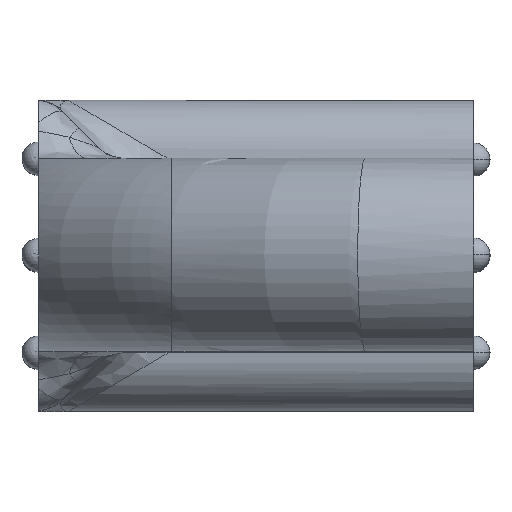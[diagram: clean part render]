
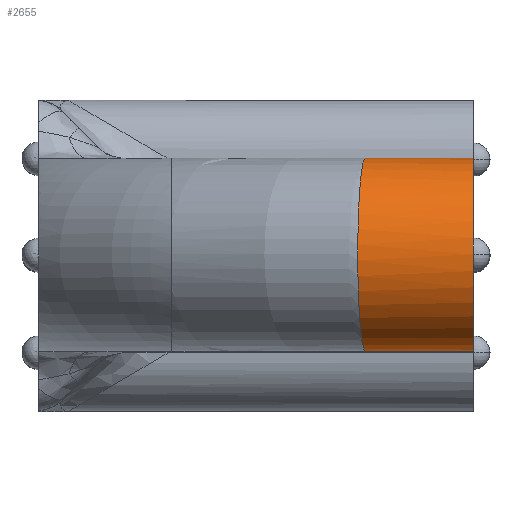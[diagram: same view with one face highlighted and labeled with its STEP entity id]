
A CAD part, top view. The second image highlights one B-rep face of the part: STEP entity #2655.
In plain terms, the highlighted cylindrical face has radius 11.509 mm (diameter 23.019 mm), a partial arc.
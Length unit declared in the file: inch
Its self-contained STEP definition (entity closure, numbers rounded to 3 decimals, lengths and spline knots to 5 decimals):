
#6 = CARTESIAN_POINT ( 'NONE',  ( 2.26457, -0.8937, 0.96371 ) ) ;
#24 = CARTESIAN_POINT ( 'NONE',  ( 1.75888, -0.8937, 0.96371 ) ) ;
#48 = DIRECTION ( 'NONE',  ( -1., 0., 0. ) ) ;
#53 = CARTESIAN_POINT ( 'NONE',  ( 8.36796, -0.8937, 0.96371 ) ) ;
#144 = CIRCLE ( 'NONE', #2152, 0.45313 ) ;
#151 = VECTOR ( 'NONE', #2381, 39.37008 ) ;
#177 = LINE ( 'NONE', #2359, #151 ) ;
#347 = CYLINDRICAL_SURFACE ( 'NONE', #2343, 0.45313 ) ;
#355 = FACE_OUTER_BOUND ( 'NONE', #2465, .T. ) ;
#608 = LINE ( 'NONE', #53, #613 ) ;
#613 = VECTOR ( 'NONE', #48, 39.37008 ) ;
#1392 = CARTESIAN_POINT ( 'NONE',  ( 1.75888, -1.79995, 0.96371 ) ) ;
#1609 = EDGE_CURVE ( 'NONE', #1746, #1688, #608, .T. ) ;
#1688 = VERTEX_POINT ( 'NONE', #24 ) ;
#1746 = VERTEX_POINT ( 'NONE', #6 ) ;
#1852 = VERTEX_POINT ( 'NONE', #3689 ) ;
#1872 = CARTESIAN_POINT ( 'NONE',  ( 1.75888, -1.79995, 0.96371 ) ) ;
#1876 = CARTESIAN_POINT ( 'NONE',  ( 1.75826, -1.79995, 0.97107 ) ) ;
#1880 = CARTESIAN_POINT ( 'NONE',  ( 1.75762, -1.79976, 0.97861 ) ) ;
#1885 = CARTESIAN_POINT ( 'NONE',  ( 1.75636, -1.79903, 0.99351 ) ) ;
#1889 = CARTESIAN_POINT ( 'NONE',  ( 1.75573, -1.79848, 1.00096 ) ) ;
#1890 = CARTESIAN_POINT ( 'NONE',  ( 1.75385, -1.79627, 1.02325 ) ) ;
#1895 = CARTESIAN_POINT ( 'NONE',  ( 1.75262, -1.79407, 1.03793 ) ) ;
#1901 = CARTESIAN_POINT ( 'NONE',  ( 1.74901, -1.7854, 1.08138 ) ) ;
#1902 = CARTESIAN_POINT ( 'NONE',  ( 1.74669, -1.77685, 1.10959 ) ) ;
#1906 = CARTESIAN_POINT ( 'NONE',  ( 1.74333, -1.75981, 1.15074 ) ) ;
#1908 = CARTESIAN_POINT ( 'NONE',  ( 1.74223, -1.75339, 1.16431 ) ) ;
#1915 = CARTESIAN_POINT ( 'NONE',  ( 1.74011, -1.7394, 1.19049 ) ) ;
#1916 = CARTESIAN_POINT ( 'NONE',  ( 1.73909, -1.73179, 1.20316 ) ) ;
#1921 = CARTESIAN_POINT ( 'NONE',  ( 1.73614, -1.70721, 1.23996 ) ) ;
#1922 = CARTESIAN_POINT ( 'NONE',  ( 1.73432, -1.68841, 1.26293 ) ) ;
#1929 = CARTESIAN_POINT ( 'NONE',  ( 1.73098, -1.64615, 1.30521 ) ) ;
#1933 = CARTESIAN_POINT ( 'NONE',  ( 1.72951, -1.62327, 1.32395 ) ) ;
#1935 = CARTESIAN_POINT ( 'NONE',  ( 1.72759, -1.58642, 1.34859 ) ) ;
#1944 = CARTESIAN_POINT ( 'NONE',  ( 1.727, -1.57371, 1.35622 ) ) ;
#1945 = CARTESIAN_POINT ( 'NONE',  ( 1.72591, -1.54742, 1.37029 ) ) ;
#1949 = CARTESIAN_POINT ( 'NONE',  ( 1.72541, -1.53384, 1.37671 ) ) ;
#1952 = CARTESIAN_POINT ( 'NONE',  ( 1.72409, -1.49267, 1.39375 ) ) ;
#1956 = CARTESIAN_POINT ( 'NONE',  ( 1.72343, -1.46439, 1.40232 ) ) ;
#1961 = CARTESIAN_POINT ( 'NONE',  ( 1.72277, -1.42071, 1.41102 ) ) ;
#1962 = CARTESIAN_POINT ( 'NONE',  ( 1.7226, -1.40586, 1.41322 ) ) ;
#1968 = CARTESIAN_POINT ( 'NONE',  ( 1.72237, -1.37614, 1.41613 ) ) ;
#1969 = CARTESIAN_POINT ( 'NONE',  ( 1.72232, -1.36132, 1.41684 ) ) ;
#1974 = CARTESIAN_POINT ( 'NONE',  ( 1.72232, -1.31693, 1.41682 ) ) ;
#1977 = CARTESIAN_POINT ( 'NONE',  ( 1.72254, -1.28748, 1.41393 ) ) ;
#1979 = CARTESIAN_POINT ( 'NONE',  ( 1.72322, -1.24349, 1.40515 ) ) ;
#1983 = CARTESIAN_POINT ( 'NONE',  ( 1.7235, -1.22897, 1.40149 ) ) ;
#1984 = CARTESIAN_POINT ( 'NONE',  ( 1.72416, -1.2006, 1.39285 ) ) ;
#1988 = CARTESIAN_POINT ( 'NONE',  ( 1.72494, -1.17277, 1.38285 ) ) ;
#1990 = CARTESIAN_POINT ( 'NONE',  ( 1.72592, -1.14602, 1.37019 ) ) ;
#1992 = CARTESIAN_POINT ( 'NONE',  ( 1.727, -1.11983, 1.35616 ) ) ;
#1995 = CARTESIAN_POINT ( 'NONE',  ( 1.72761, -1.10694, 1.34842 ) ) ;
#1996 = CARTESIAN_POINT ( 'NONE',  ( 1.72955, -1.06983, 1.32355 ) ) ;
#2001 = CARTESIAN_POINT ( 'NONE',  ( 1.73102, -1.04704, 1.30478 ) ) ;
#2006 = CARTESIAN_POINT ( 'NONE',  ( 1.73432, -1.00525, 1.26292 ) ) ;
#2007 = CARTESIAN_POINT ( 'NONE',  ( 1.73617, -0.98613, 1.23958 ) ) ;
#2010 = CARTESIAN_POINT ( 'NONE',  ( 1.74012, -0.95334, 1.19035 ) ) ;
#2011 = CARTESIAN_POINT ( 'NONE',  ( 1.74222, -0.93945, 1.16434 ) ) ;
#2020 = CARTESIAN_POINT ( 'NONE',  ( 1.74558, -0.92243, 1.12319 ) ) ;
#2022 = CARTESIAN_POINT ( 'NONE',  ( 1.74673, -0.91739, 1.10906 ) ) ;
#2026 = CARTESIAN_POINT ( 'NONE',  ( 1.74907, -0.9088, 1.08065 ) ) ;
#2029 = CARTESIAN_POINT ( 'NONE',  ( 1.75026, -0.90522, 1.06632 ) ) ;
#2036 = CARTESIAN_POINT ( 'NONE',  ( 1.75267, -0.89949, 1.03742 ) ) ;
#2038 = CARTESIAN_POINT ( 'NONE',  ( 1.75389, -0.89733, 1.02284 ) ) ;
#2046 = CARTESIAN_POINT ( 'NONE',  ( 1.75574, -0.89516, 1.0008 ) ) ;
#2049 = CARTESIAN_POINT ( 'NONE',  ( 1.75636, -0.89461, 0.99342 ) ) ;
#2051 = CARTESIAN_POINT ( 'NONE',  ( 1.75762, -0.89388, 0.9786 ) ) ;
#2054 = CARTESIAN_POINT ( 'NONE',  ( 1.75826, -0.8937, 0.97107 ) ) ;
#2057 = CARTESIAN_POINT ( 'NONE',  ( 1.75888, -0.8937, 0.96371 ) ) ;
#2120 = DIRECTION ( 'NONE',  ( 0., -1., 0. ) ) ;
#2123 = DIRECTION ( 'NONE',  ( 1., 0., 0. ) ) ;
#2128 = CARTESIAN_POINT ( 'NONE',  ( 2.26457, -1.34682, 0.96371 ) ) ;
#2152 = AXIS2_PLACEMENT_3D ( 'NONE', #2128, #2123, #2120 ) ;
#2179 = ORIENTED_EDGE ( 'NONE', *, *, #3055, .F. ) ;
#2190 = ORIENTED_EDGE ( 'NONE', *, *, #1609, .T. ) ;
#2202 = ORIENTED_EDGE ( 'NONE', *, *, #3069, .T. ) ;
#2220 = ORIENTED_EDGE ( 'NONE', *, *, #2939, .F. ) ;
#2343 = AXIS2_PLACEMENT_3D ( 'NONE', #2419, #2410, #2402 ) ;
#2359 = CARTESIAN_POINT ( 'NONE',  ( 8.36796, -1.79995, 0.96371 ) ) ;
#2381 = DIRECTION ( 'NONE',  ( -1., 0., 0. ) ) ;
#2402 = DIRECTION ( 'NONE',  ( 0., 1., 0. ) ) ;
#2410 = DIRECTION ( 'NONE',  ( -1., 0., 0. ) ) ;
#2419 = CARTESIAN_POINT ( 'NONE',  ( 8.36796, -1.34682, 0.96371 ) ) ;
#2465 = EDGE_LOOP ( 'NONE', ( #2179, #2190, #2202, #2220 ) ) ;
#2655 = ADVANCED_FACE ( 'NONE', ( #355 ), #347, .T. ) ;
#2808 = B_SPLINE_CURVE_WITH_KNOTS ( 'NONE', 3,
 ( #2057, #2054, #2051, #2049, #2046, #2038, #2036, #2029, #2026, #2022, #2020, #2011, #2010, #2007, #2006, #2001, #1996, #1995, #1992, #1990, #1988, #1984, #1983, #1979, #1977, #1974, #1969, #1968, #1962, #1961, #1956, #1952, #1949, #1945, #1944, #1935, #1933, #1929, #1922, #1921, #1916, #1915, #1908, #1906, #1902, #1901, #1895, #1890, #1889, #1885, #1880, #1876, #1872 ),
 .UNSPECIFIED., .F., .F.,
 ( 4, 2, 2, 2, 2, 2, 2, 2, 2, 2, 1, 2, 2, 2, 2, 2, 2, 2, 2, 2, 2, 2, 2, 2, 2, 2, 4 ),
 ( -0.00005, 0.00051, 0.00107, 0.0022, 0.00333, 0.00445, 0.0067, 0.00896, 0.01121, 0.01234, 0.01346, 0.01459, 0.01571, 0.01797, 0.01909, 0.02022, 0.02247, 0.0236, 0.02472, 0.02697, 0.02923, 0.03035, 0.03148, 0.03373, 0.03486, 0.03542, 0.03598 ),
 .UNSPECIFIED. ) ;
#2939 = EDGE_CURVE ( 'NONE', #1852, #3293, #177, .T. ) ;
#3055 = EDGE_CURVE ( 'NONE', #1746, #1852, #144, .T. ) ;
#3069 = EDGE_CURVE ( 'NONE', #1688, #3293, #2808, .T. ) ;
#3293 = VERTEX_POINT ( 'NONE', #1392 ) ;
#3689 = CARTESIAN_POINT ( 'NONE',  ( 2.26457, -1.79995, 0.96371 ) ) ;
